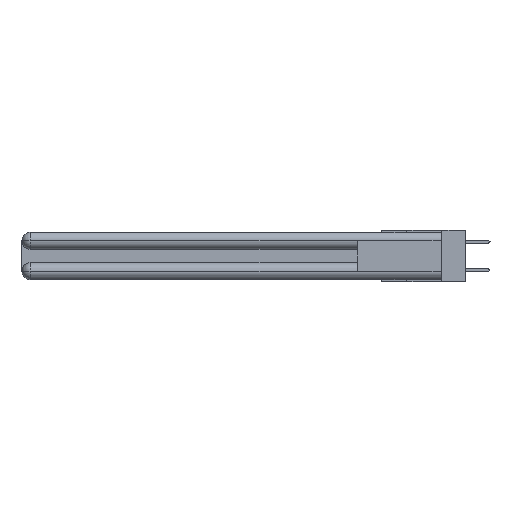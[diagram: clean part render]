
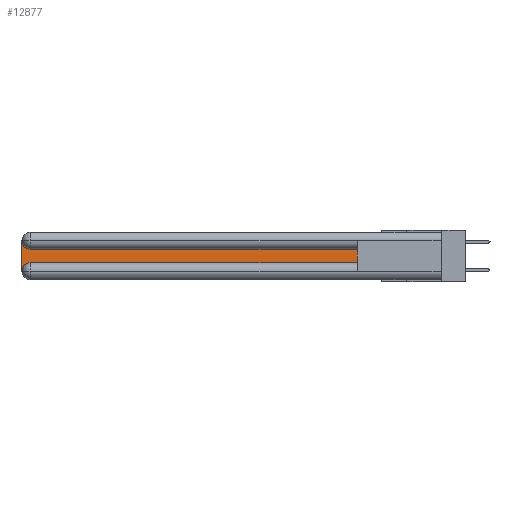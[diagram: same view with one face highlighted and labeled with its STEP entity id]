
A CAD part, left-side view. The second image highlights one B-rep face of the part: STEP entity #12877.
In plain terms, the highlighted planar face has unit normal (-1, 0, 0).
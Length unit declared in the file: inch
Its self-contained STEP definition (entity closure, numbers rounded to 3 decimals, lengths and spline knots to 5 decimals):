
#1071 = VECTOR ( 'NONE', #14225, 39.37008 ) ;
#2423 = VERTEX_POINT ( 'NONE', #5241 ) ;
#3035 = CARTESIAN_POINT ( 'NONE',  ( 0.075, 3., -0.2175 ) ) ;
#3132 = CARTESIAN_POINT ( 'NONE',  ( 0.075, 0.6, -0.1225 ) ) ;
#3883 = DIRECTION ( 'NONE',  ( 0., -1., 0. ) ) ;
#4013 = PLANE ( 'NONE',  #30621 ) ;
#4243 = CARTESIAN_POINT ( 'NONE',  ( 0.075, 3., -0.1225 ) ) ;
#5241 = CARTESIAN_POINT ( 'NONE',  ( 0.075, 2.94, -0.2175 ) ) ;
#5567 = DIRECTION ( 'NONE',  ( 0., 1., 0. ) ) ;
#5853 = VECTOR ( 'NONE', #3883, 39.37008 ) ;
#6509 = EDGE_CURVE ( 'NONE', #6659, #25001, #10513, .T. ) ;
#6583 = LINE ( 'NONE', #3132, #31858 ) ;
#6659 = VERTEX_POINT ( 'NONE', #8877 ) ;
#6664 = ORIENTED_EDGE ( 'NONE', *, *, #13919, .T. ) ;
#6723 = CARTESIAN_POINT ( 'NONE',  ( 0.075, 0.6, -0.2175 ) ) ;
#6961 = EDGE_CURVE ( 'NONE', #35763, #6659, #6583, .T. ) ;
#7673 = FACE_OUTER_BOUND ( 'NONE', #12315, .T. ) ;
#8060 = CARTESIAN_POINT ( 'NONE',  ( 0.075, 2.94, -0.2775 ) ) ;
#8877 = CARTESIAN_POINT ( 'NONE',  ( 0.075, 2.94, -0.1225 ) ) ;
#9551 = AXIS2_PLACEMENT_3D ( 'NONE', #8060, #22208, #33065 ) ;
#10513 = CIRCLE ( 'NONE', #19472, 0.06 ) ;
#11004 = CARTESIAN_POINT ( 'NONE',  ( 0.075, 3., -0.0625 ) ) ;
#11553 = EDGE_CURVE ( 'NONE', #16974, #2423, #21258, .T. ) ;
#12315 = EDGE_LOOP ( 'NONE', ( #23314, #16012, #18394, #28675, #6664, #20188 ) ) ;
#12877 = ADVANCED_FACE ( 'NONE', ( #7673 ), #4013, .F. ) ;
#13264 = EDGE_CURVE ( 'NONE', #25001, #16974, #23761, .T. ) ;
#13761 = DIRECTION ( 'NONE',  ( 0., 0., -1. ) ) ;
#13919 = EDGE_CURVE ( 'NONE', #2423, #18183, #16761, .T. ) ;
#14225 = DIRECTION ( 'NONE',  ( 0., 0., -1. ) ) ;
#14604 = CARTESIAN_POINT ( 'NONE',  ( 0.075, 0.6, -0.2175 ) ) ;
#14956 = DIRECTION ( 'NONE',  ( 0., 0., -1. ) ) ;
#15765 = CARTESIAN_POINT ( 'NONE',  ( 0.075, 3., -0.2775 ) ) ;
#16012 = ORIENTED_EDGE ( 'NONE', *, *, #6509, .T. ) ;
#16761 = LINE ( 'NONE', #14604, #5853 ) ;
#16974 = VERTEX_POINT ( 'NONE', #15765 ) ;
#18183 = VERTEX_POINT ( 'NONE', #24903 ) ;
#18394 = ORIENTED_EDGE ( 'NONE', *, *, #13264, .T. ) ;
#19472 = AXIS2_PLACEMENT_3D ( 'NONE', #27882, #19775, #13761 ) ;
#19494 = LINE ( 'NONE', #6723, #27745 ) ;
#19775 = DIRECTION ( 'NONE',  ( 1., 0., 0. ) ) ;
#20188 = ORIENTED_EDGE ( 'NONE', *, *, #22091, .T. ) ;
#20544 = DIRECTION ( 'NONE',  ( 0., 0., 1. ) ) ;
#21258 = CIRCLE ( 'NONE', #9551, 0.06 ) ;
#22091 = EDGE_CURVE ( 'NONE', #18183, #35763, #19494, .T. ) ;
#22208 = DIRECTION ( 'NONE',  ( 1., 0., 0. ) ) ;
#22410 = CARTESIAN_POINT ( 'NONE',  ( 0.075, 0.6, -0.1225 ) ) ;
#23245 = DIRECTION ( 'NONE',  ( 1., 0., 0. ) ) ;
#23314 = ORIENTED_EDGE ( 'NONE', *, *, #6961, .T. ) ;
#23761 = LINE ( 'NONE', #3035, #1071 ) ;
#24903 = CARTESIAN_POINT ( 'NONE',  ( 0.075, 0.6, -0.2175 ) ) ;
#25001 = VERTEX_POINT ( 'NONE', #11004 ) ;
#27745 = VECTOR ( 'NONE', #20544, 39.37008 ) ;
#27882 = CARTESIAN_POINT ( 'NONE',  ( 0.075, 2.94, -0.0625 ) ) ;
#28675 = ORIENTED_EDGE ( 'NONE', *, *, #11553, .T. ) ;
#30621 = AXIS2_PLACEMENT_3D ( 'NONE', #4243, #23245, #14956 ) ;
#31858 = VECTOR ( 'NONE', #5567, 39.37008 ) ;
#33065 = DIRECTION ( 'NONE',  ( 0., 0., -1. ) ) ;
#35763 = VERTEX_POINT ( 'NONE', #22410 ) ;
